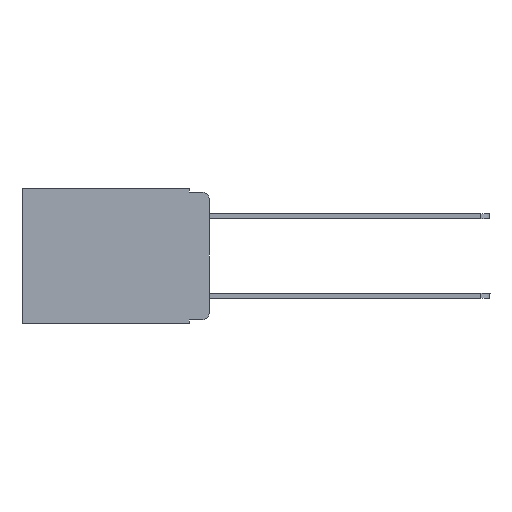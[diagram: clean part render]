
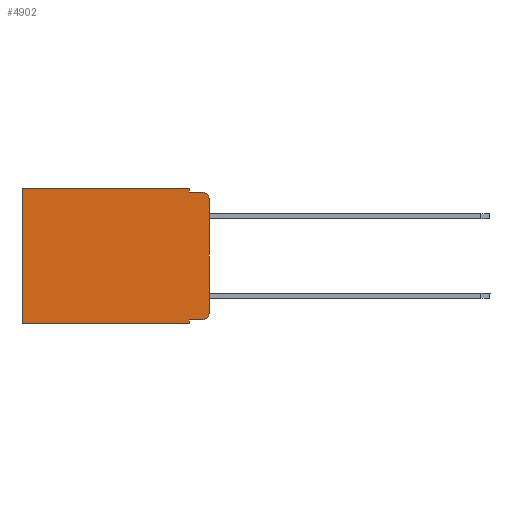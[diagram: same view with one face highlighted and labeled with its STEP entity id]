
A CAD part, left-side view. The second image highlights one B-rep face of the part: STEP entity #4902.
In plain terms, the highlighted planar face has unit normal (-1, 0, 0).
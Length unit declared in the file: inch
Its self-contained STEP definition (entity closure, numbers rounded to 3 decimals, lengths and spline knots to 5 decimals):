
#200 = ORIENTED_EDGE ( 'NONE', *, *, #2955, .T. ) ;
#306 = CARTESIAN_POINT ( 'NONE',  ( 0.298, 0.473, 0. ) ) ;
#481 = DIRECTION ( 'NONE',  ( -1., 0., 0. ) ) ;
#897 = VERTEX_POINT ( 'NONE', #19557 ) ;
#967 = VERTEX_POINT ( 'NONE', #2621 ) ;
#1202 = ORIENTED_EDGE ( 'NONE', *, *, #6817, .F. ) ;
#1484 = DIRECTION ( 'NONE',  ( 1., 0., 0. ) ) ;
#1604 = DIRECTION ( 'NONE',  ( 0., 0., -1. ) ) ;
#1729 = EDGE_CURVE ( 'NONE', #897, #14476, #10544, .T. ) ;
#1746 = EDGE_LOOP ( 'NONE', ( #13956, #11436, #15679, #1202, #18936, #200, #20063, #20635, #20902, #5709 ) ) ;
#2356 = VECTOR ( 'NONE', #13748, 39.37008 ) ;
#2621 = CARTESIAN_POINT ( 'NONE',  ( 0.298, 0.051, -0.01 ) ) ;
#2742 = VECTOR ( 'NONE', #1604, 39.37008 ) ;
#2955 = EDGE_CURVE ( 'NONE', #10761, #21733, #10198, .T. ) ;
#3350 = CARTESIAN_POINT ( 'NONE',  ( 0.298, 0.473, -0.343 ) ) ;
#4074 = DIRECTION ( 'NONE',  ( 0., -1., 0. ) ) ;
#4110 = CARTESIAN_POINT ( 'NONE',  ( 0.298, 0.02, -0.01 ) ) ;
#4220 = DIRECTION ( 'NONE',  ( 0., 1., 0. ) ) ;
#4526 = EDGE_CURVE ( 'NONE', #7928, #14476, #11719, .T. ) ;
#4595 = EDGE_CURVE ( 'NONE', #13034, #10761, #18727, .T. ) ;
#4634 = VECTOR ( 'NONE', #4220, 39.37008 ) ;
#4902 = ADVANCED_FACE ( 'NONE', ( #19585 ), #5337, .F. ) ;
#5337 = PLANE ( 'NONE',  #17446 ) ;
#5435 = CARTESIAN_POINT ( 'NONE',  ( 0.298, 0.02, -0.333 ) ) ;
#5576 = DIRECTION ( 'NONE',  ( 0., 0., -1. ) ) ;
#5709 = ORIENTED_EDGE ( 'NONE', *, *, #4526, .T. ) ;
#5876 = DIRECTION ( 'NONE',  ( 0., 0., -1. ) ) ;
#6354 = CARTESIAN_POINT ( 'NONE',  ( 0.298, 0.02, -0.313 ) ) ;
#6776 = CARTESIAN_POINT ( 'NONE',  ( 0.298, 0.051, -0.333 ) ) ;
#6817 = EDGE_CURVE ( 'NONE', #13034, #967, #18863, .T. ) ;
#7442 = VERTEX_POINT ( 'NONE', #6776 ) ;
#7625 = DIRECTION ( 'NONE',  ( 0., -1., 0. ) ) ;
#7928 = VERTEX_POINT ( 'NONE', #5435 ) ;
#8016 = EDGE_CURVE ( 'NONE', #897, #22876, #18969, .T. ) ;
#8229 = CARTESIAN_POINT ( 'NONE',  ( 0.298, 0., -0.313 ) ) ;
#9727 = CARTESIAN_POINT ( 'NONE',  ( 0.298, 0.051, -0.333 ) ) ;
#9865 = CARTESIAN_POINT ( 'NONE',  ( 0.298, 0., 0. ) ) ;
#10198 = LINE ( 'NONE', #17389, #2356 ) ;
#10476 = LINE ( 'NONE', #17665, #16763 ) ;
#10544 = LINE ( 'NONE', #21144, #2742 ) ;
#10761 = VERTEX_POINT ( 'NONE', #306 ) ;
#11209 = CARTESIAN_POINT ( 'NONE',  ( 0.298, 0.051, 0. ) ) ;
#11436 = ORIENTED_EDGE ( 'NONE', *, *, #8016, .T. ) ;
#11719 = CIRCLE ( 'NONE', #19619, 0.02 ) ;
#12166 = CARTESIAN_POINT ( 'NONE',  ( 0.298, 0., 0. ) ) ;
#13034 = VERTEX_POINT ( 'NONE', #11209 ) ;
#13748 = DIRECTION ( 'NONE',  ( 0., 0., -1. ) ) ;
#13845 = DIRECTION ( 'NONE',  ( 0., 0., -1. ) ) ;
#13956 = ORIENTED_EDGE ( 'NONE', *, *, #1729, .F. ) ;
#14476 = VERTEX_POINT ( 'NONE', #8229 ) ;
#14756 = LINE ( 'NONE', #16288, #18254 ) ;
#14816 = CARTESIAN_POINT ( 'NONE',  ( 0.298, 0., -0.343 ) ) ;
#14994 = DIRECTION ( 'NONE',  ( 0., 0., -1. ) ) ;
#15679 = ORIENTED_EDGE ( 'NONE', *, *, #22725, .F. ) ;
#16241 = EDGE_CURVE ( 'NONE', #22769, #21733, #16474, .T. ) ;
#16288 = CARTESIAN_POINT ( 'NONE',  ( 0.298, 0.051, 0. ) ) ;
#16474 = LINE ( 'NONE', #14816, #22461 ) ;
#16763 = VECTOR ( 'NONE', #7625, 39.37008 ) ;
#17018 = LINE ( 'NONE', #9727, #19065 ) ;
#17051 = EDGE_CURVE ( 'NONE', #7442, #22769, #14756, .T. ) ;
#17085 = DIRECTION ( 'NONE',  ( 0., 0., -1. ) ) ;
#17389 = CARTESIAN_POINT ( 'NONE',  ( 0.298, 0.473, 0. ) ) ;
#17446 = AXIS2_PLACEMENT_3D ( 'NONE', #12166, #1484, #13845 ) ;
#17665 = CARTESIAN_POINT ( 'NONE',  ( 0.298, 0.051, -0.01 ) ) ;
#17834 = AXIS2_PLACEMENT_3D ( 'NONE', #19930, #481, #14994 ) ;
#18117 = VECTOR ( 'NONE', #17085, 39.37008 ) ;
#18254 = VECTOR ( 'NONE', #5576, 39.37008 ) ;
#18727 = LINE ( 'NONE', #9865, #4634 ) ;
#18863 = LINE ( 'NONE', #22515, #18117 ) ;
#18936 = ORIENTED_EDGE ( 'NONE', *, *, #4595, .T. ) ;
#18969 = CIRCLE ( 'NONE', #17834, 0.02 ) ;
#19065 = VECTOR ( 'NONE', #4074, 39.37008 ) ;
#19557 = CARTESIAN_POINT ( 'NONE',  ( 0.298, 0., -0.03 ) ) ;
#19585 = FACE_OUTER_BOUND ( 'NONE', #1746, .T. ) ;
#19619 = AXIS2_PLACEMENT_3D ( 'NONE', #6354, #20463, #5876 ) ;
#19686 = EDGE_CURVE ( 'NONE', #7442, #7928, #17018, .T. ) ;
#19930 = CARTESIAN_POINT ( 'NONE',  ( 0.298, 0.02, -0.03 ) ) ;
#20063 = ORIENTED_EDGE ( 'NONE', *, *, #16241, .F. ) ;
#20117 = CARTESIAN_POINT ( 'NONE',  ( 0.298, 0.051, -0.343 ) ) ;
#20463 = DIRECTION ( 'NONE',  ( -1., 0., 0. ) ) ;
#20635 = ORIENTED_EDGE ( 'NONE', *, *, #17051, .F. ) ;
#20902 = ORIENTED_EDGE ( 'NONE', *, *, #19686, .T. ) ;
#21144 = CARTESIAN_POINT ( 'NONE',  ( 0.298, 0., 0. ) ) ;
#21733 = VERTEX_POINT ( 'NONE', #3350 ) ;
#21875 = DIRECTION ( 'NONE',  ( 0., 1., 0. ) ) ;
#22461 = VECTOR ( 'NONE', #21875, 39.37008 ) ;
#22515 = CARTESIAN_POINT ( 'NONE',  ( 0.298, 0.051, 0. ) ) ;
#22725 = EDGE_CURVE ( 'NONE', #967, #22876, #10476, .T. ) ;
#22769 = VERTEX_POINT ( 'NONE', #20117 ) ;
#22876 = VERTEX_POINT ( 'NONE', #4110 ) ;
